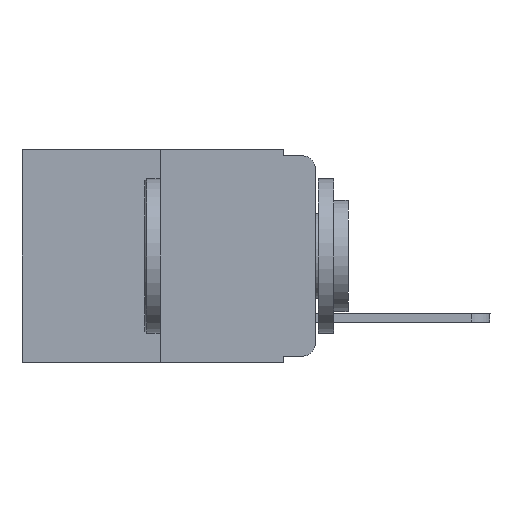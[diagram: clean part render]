
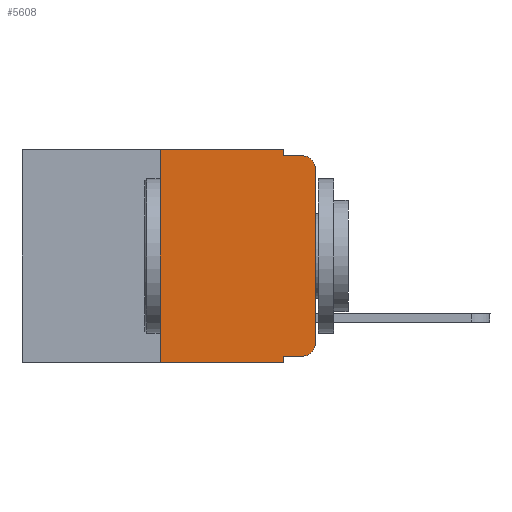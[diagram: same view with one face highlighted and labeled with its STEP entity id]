
A CAD part, left-side view. The second image highlights one B-rep face of the part: STEP entity #5608.
In plain terms, the highlighted planar face has unit normal (-1, 0, 0).
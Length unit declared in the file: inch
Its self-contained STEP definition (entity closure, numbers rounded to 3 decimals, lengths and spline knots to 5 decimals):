
#124 = EDGE_LOOP ( 'NONE', ( #12776, #8488, #12189, #8325, #16867, #10622, #18687, #8099, #5783, #4089 ) ) ;
#337 = CARTESIAN_POINT ( 'NONE',  ( 0., 0.051, 0. ) ) ;
#663 = CARTESIAN_POINT ( 'NONE',  ( 0., 0.25, 0. ) ) ;
#780 = VERTEX_POINT ( 'NONE', #6176 ) ;
#1499 = LINE ( 'NONE', #8165, #9915 ) ;
#1559 = EDGE_CURVE ( 'NONE', #10689, #4363, #11149, .T. ) ;
#1766 = DIRECTION ( 'NONE',  ( 0., 0., 1. ) ) ;
#2168 = DIRECTION ( 'NONE',  ( 1., 0., 0. ) ) ;
#2383 = PLANE ( 'NONE',  #5026 ) ;
#2869 = VERTEX_POINT ( 'NONE', #4179 ) ;
#3067 = CARTESIAN_POINT ( 'NONE',  ( 0., 0.02, -0.03 ) ) ;
#3338 = VECTOR ( 'NONE', #8117, 39.37008 ) ;
#4089 = ORIENTED_EDGE ( 'NONE', *, *, #14608, .T. ) ;
#4179 = CARTESIAN_POINT ( 'NONE',  ( 0., 0., -0.03 ) ) ;
#4363 = VERTEX_POINT ( 'NONE', #5564 ) ;
#5026 = AXIS2_PLACEMENT_3D ( 'NONE', #12669, #2168, #19338 ) ;
#5063 = CIRCLE ( 'NONE', #18043, 0.02 ) ;
#5189 = CARTESIAN_POINT ( 'NONE',  ( 0., 0.25, -0.343 ) ) ;
#5437 = VERTEX_POINT ( 'NONE', #10496 ) ;
#5564 = CARTESIAN_POINT ( 'NONE',  ( 0., 0.051, 0. ) ) ;
#5608 = ADVANCED_FACE ( 'NONE', ( #19142 ), #2383, .F. ) ;
#5719 = VERTEX_POINT ( 'NONE', #19567 ) ;
#5783 = ORIENTED_EDGE ( 'NONE', *, *, #7031, .T. ) ;
#6176 = CARTESIAN_POINT ( 'NONE',  ( 0., 0.051, -0.01 ) ) ;
#6203 = DIRECTION ( 'NONE',  ( 0., 0., -1. ) ) ;
#6336 = CARTESIAN_POINT ( 'NONE',  ( 0., 0., -0.313 ) ) ;
#6736 = DIRECTION ( 'NONE',  ( -1., 0., 0. ) ) ;
#6813 = LINE ( 'NONE', #13509, #3338 ) ;
#7031 = EDGE_CURVE ( 'NONE', #5719, #11028, #1499, .T. ) ;
#7113 = CARTESIAN_POINT ( 'NONE',  ( 0., 0., 0. ) ) ;
#7477 = LINE ( 'NONE', #14184, #12927 ) ;
#7961 = CARTESIAN_POINT ( 'NONE',  ( 0., 0.051, 0. ) ) ;
#8030 = VERTEX_POINT ( 'NONE', #6336 ) ;
#8099 = ORIENTED_EDGE ( 'NONE', *, *, #12300, .F. ) ;
#8117 = DIRECTION ( 'NONE',  ( 0., -1., 0. ) ) ;
#8165 = CARTESIAN_POINT ( 'NONE',  ( 0., 0.051, -0.333 ) ) ;
#8325 = ORIENTED_EDGE ( 'NONE', *, *, #15736, .F. ) ;
#8488 = ORIENTED_EDGE ( 'NONE', *, *, #10408, .T. ) ;
#9503 = DIRECTION ( 'NONE',  ( 0., -1., 0. ) ) ;
#9608 = CARTESIAN_POINT ( 'NONE',  ( 0., 0.473, 0. ) ) ;
#9694 = CIRCLE ( 'NONE', #11102, 0.02 ) ;
#9915 = VECTOR ( 'NONE', #17490, 39.37008 ) ;
#10180 = DIRECTION ( 'NONE',  ( 0., 0., -1. ) ) ;
#10271 = VERTEX_POINT ( 'NONE', #5189 ) ;
#10288 = LINE ( 'NONE', #337, #11797 ) ;
#10408 = EDGE_CURVE ( 'NONE', #2869, #5437, #5063, .T. ) ;
#10496 = CARTESIAN_POINT ( 'NONE',  ( 0., 0.02, -0.01 ) ) ;
#10622 = ORIENTED_EDGE ( 'NONE', *, *, #18994, .F. ) ;
#10689 = VERTEX_POINT ( 'NONE', #663 ) ;
#10715 = VERTEX_POINT ( 'NONE', #17424 ) ;
#11028 = VERTEX_POINT ( 'NONE', #18273 ) ;
#11102 = AXIS2_PLACEMENT_3D ( 'NONE', #19891, #6736, #18259 ) ;
#11149 = LINE ( 'NONE', #9608, #12926 ) ;
#11797 = VECTOR ( 'NONE', #10180, 39.37008 ) ;
#11820 = CARTESIAN_POINT ( 'NONE',  ( 0., 0.25, 0. ) ) ;
#12189 = ORIENTED_EDGE ( 'NONE', *, *, #16403, .F. ) ;
#12300 = EDGE_CURVE ( 'NONE', #5719, #10715, #10288, .T. ) ;
#12669 = CARTESIAN_POINT ( 'NONE',  ( 0., 0.473, 0. ) ) ;
#12776 = ORIENTED_EDGE ( 'NONE', *, *, #13666, .T. ) ;
#12829 = DIRECTION ( 'NONE',  ( -1., 0., 0. ) ) ;
#12926 = VECTOR ( 'NONE', #9503, 39.37008 ) ;
#12927 = VECTOR ( 'NONE', #19098, 39.37008 ) ;
#13349 = LINE ( 'NONE', #11820, #19751 ) ;
#13509 = CARTESIAN_POINT ( 'NONE',  ( 0., 0.473, -0.343 ) ) ;
#13666 = EDGE_CURVE ( 'NONE', #8030, #2869, #20161, .T. ) ;
#14184 = CARTESIAN_POINT ( 'NONE',  ( 0., 0.051, -0.01 ) ) ;
#14608 = EDGE_CURVE ( 'NONE', #11028, #8030, #9694, .T. ) ;
#15736 = EDGE_CURVE ( 'NONE', #4363, #780, #18065, .T. ) ;
#16113 = DIRECTION ( 'NONE',  ( 0., 0., -1. ) ) ;
#16403 = EDGE_CURVE ( 'NONE', #780, #5437, #7477, .T. ) ;
#16525 = DIRECTION ( 'NONE',  ( 0., 0., 1. ) ) ;
#16728 = EDGE_CURVE ( 'NONE', #10271, #10715, #6813, .T. ) ;
#16867 = ORIENTED_EDGE ( 'NONE', *, *, #1559, .F. ) ;
#17079 = VECTOR ( 'NONE', #1766, 39.37008 ) ;
#17424 = CARTESIAN_POINT ( 'NONE',  ( 0., 0.051, -0.343 ) ) ;
#17490 = DIRECTION ( 'NONE',  ( 0., -1., 0. ) ) ;
#17797 = VECTOR ( 'NONE', #6203, 39.37008 ) ;
#18043 = AXIS2_PLACEMENT_3D ( 'NONE', #3067, #12829, #16113 ) ;
#18065 = LINE ( 'NONE', #7961, #17797 ) ;
#18259 = DIRECTION ( 'NONE',  ( 0., 0., -1. ) ) ;
#18273 = CARTESIAN_POINT ( 'NONE',  ( 0., 0.02, -0.333 ) ) ;
#18687 = ORIENTED_EDGE ( 'NONE', *, *, #16728, .T. ) ;
#18994 = EDGE_CURVE ( 'NONE', #10271, #10689, #13349, .T. ) ;
#19098 = DIRECTION ( 'NONE',  ( 0., -1., 0. ) ) ;
#19142 = FACE_OUTER_BOUND ( 'NONE', #124, .T. ) ;
#19338 = DIRECTION ( 'NONE',  ( 0., 0., -1. ) ) ;
#19567 = CARTESIAN_POINT ( 'NONE',  ( 0., 0.051, -0.333 ) ) ;
#19751 = VECTOR ( 'NONE', #16525, 39.37008 ) ;
#19891 = CARTESIAN_POINT ( 'NONE',  ( 0., 0.02, -0.313 ) ) ;
#20161 = LINE ( 'NONE', #7113, #17079 ) ;
